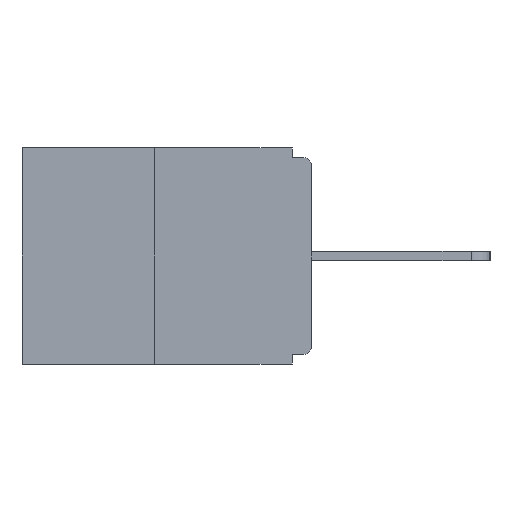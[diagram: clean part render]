
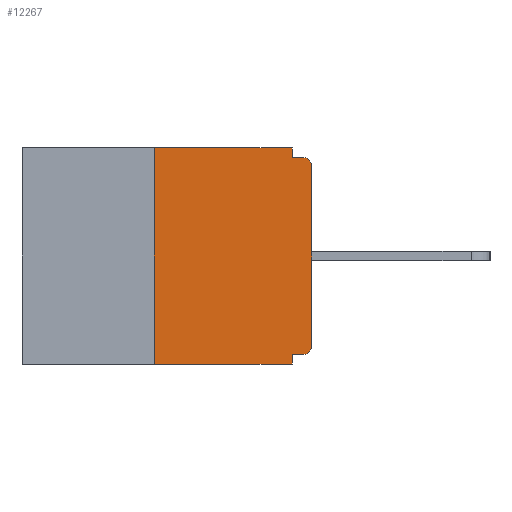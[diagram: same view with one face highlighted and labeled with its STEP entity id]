
A CAD part, left-side view. The second image highlights one B-rep face of the part: STEP entity #12267.
In plain terms, the highlighted planar face has unit normal (-1, 0, 0).
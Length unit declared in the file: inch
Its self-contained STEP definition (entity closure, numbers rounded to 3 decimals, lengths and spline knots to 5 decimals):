
#183 = CARTESIAN_POINT ( 'NONE',  ( 0., 0.031, -0.015 ) ) ;
#197 = VERTEX_POINT ( 'NONE', #6567 ) ;
#548 = PLANE ( 'NONE',  #12446 ) ;
#624 = EDGE_CURVE ( 'NONE', #1537, #197, #9718, .T. ) ;
#679 = CARTESIAN_POINT ( 'NONE',  ( 0., 0.031, -0.328 ) ) ;
#1081 = DIRECTION ( 'NONE',  ( 0., -1., 0. ) ) ;
#1262 = ORIENTED_EDGE ( 'NONE', *, *, #9901, .F. ) ;
#1307 = DIRECTION ( 'NONE',  ( 0., 0., -1. ) ) ;
#1330 = DIRECTION ( 'NONE',  ( -1., 0., 0. ) ) ;
#1537 = VERTEX_POINT ( 'NONE', #15385 ) ;
#1835 = VERTEX_POINT ( 'NONE', #15724 ) ;
#2145 = CARTESIAN_POINT ( 'NONE',  ( 0., 0.25, -0.343 ) ) ;
#2154 = LINE ( 'NONE', #7507, #12647 ) ;
#2473 = CARTESIAN_POINT ( 'NONE',  ( 0., 0.015, -0.03 ) ) ;
#2666 = LINE ( 'NONE', #12496, #3093 ) ;
#2699 = ORIENTED_EDGE ( 'NONE', *, *, #8537, .F. ) ;
#2800 = VERTEX_POINT ( 'NONE', #5422 ) ;
#3093 = VECTOR ( 'NONE', #9903, 39.37008 ) ;
#3209 = DIRECTION ( 'NONE',  ( 0., 0., -1. ) ) ;
#3496 = DIRECTION ( 'NONE',  ( 0., 0., 1. ) ) ;
#3546 = CIRCLE ( 'NONE', #12801, 0.015 ) ;
#3568 = CARTESIAN_POINT ( 'NONE',  ( 0., 0.031, -0.343 ) ) ;
#3932 = DIRECTION ( 'NONE',  ( -1., 0., 0. ) ) ;
#4010 = ORIENTED_EDGE ( 'NONE', *, *, #9820, .F. ) ;
#4133 = ORIENTED_EDGE ( 'NONE', *, *, #13659, .F. ) ;
#4271 = EDGE_CURVE ( 'NONE', #14148, #1537, #15778, .T. ) ;
#4812 = VECTOR ( 'NONE', #1081, 39.37008 ) ;
#4949 = EDGE_LOOP ( 'NONE', ( #2699, #1262, #6456, #15787, #4010, #13012, #8579, #16400, #10294, #4133 ) ) ;
#5394 = VECTOR ( 'NONE', #3496, 39.37008 ) ;
#5422 = CARTESIAN_POINT ( 'NONE',  ( 0., 0.015, -0.328 ) ) ;
#5461 = VECTOR ( 'NONE', #8232, 39.37008 ) ;
#5687 = CARTESIAN_POINT ( 'NONE',  ( 0., 0.46, 0. ) ) ;
#6013 = CARTESIAN_POINT ( 'NONE',  ( 0., 0.25, 0. ) ) ;
#6347 = VERTEX_POINT ( 'NONE', #7987 ) ;
#6456 = ORIENTED_EDGE ( 'NONE', *, *, #12395, .T. ) ;
#6567 = CARTESIAN_POINT ( 'NONE',  ( 0., 0.015, -0.015 ) ) ;
#6991 = VERTEX_POINT ( 'NONE', #6013 ) ;
#7080 = DIRECTION ( 'NONE',  ( 0., -1., 0. ) ) ;
#7507 = CARTESIAN_POINT ( 'NONE',  ( 0., 0.46, -0.343 ) ) ;
#7617 = CARTESIAN_POINT ( 'NONE',  ( 0., 0.031, 0. ) ) ;
#7712 = VERTEX_POINT ( 'NONE', #2145 ) ;
#7987 = CARTESIAN_POINT ( 'NONE',  ( 0., 0.031, -0.343 ) ) ;
#8232 = DIRECTION ( 'NONE',  ( 0., 0., 1. ) ) ;
#8537 = EDGE_CURVE ( 'NONE', #6991, #1835, #15123, .T. ) ;
#8579 = ORIENTED_EDGE ( 'NONE', *, *, #4271, .T. ) ;
#8628 = VECTOR ( 'NONE', #15377, 39.37008 ) ;
#9718 = CIRCLE ( 'NONE', #12404, 0.015 ) ;
#9802 = CARTESIAN_POINT ( 'NONE',  ( 0., 0.46, 0. ) ) ;
#9803 = VECTOR ( 'NONE', #16550, 39.37008 ) ;
#9820 = EDGE_CURVE ( 'NONE', #2800, #10497, #2666, .T. ) ;
#9901 = EDGE_CURVE ( 'NONE', #7712, #6991, #14495, .T. ) ;
#9903 = DIRECTION ( 'NONE',  ( 0., 1., 0. ) ) ;
#10294 = ORIENTED_EDGE ( 'NONE', *, *, #16385, .F. ) ;
#10497 = VERTEX_POINT ( 'NONE', #679 ) ;
#11101 = DIRECTION ( 'NONE',  ( 1., 0., 0. ) ) ;
#11375 = CARTESIAN_POINT ( 'NONE',  ( 0., 0.25, 0. ) ) ;
#11754 = VECTOR ( 'NONE', #7080, 39.37008 ) ;
#11784 = CARTESIAN_POINT ( 'NONE',  ( 0., 0.015, -0.313 ) ) ;
#12267 = ADVANCED_FACE ( 'NONE', ( #12452 ), #548, .F. ) ;
#12395 = EDGE_CURVE ( 'NONE', #7712, #6347, #2154, .T. ) ;
#12404 = AXIS2_PLACEMENT_3D ( 'NONE', #2473, #1330, #1307 ) ;
#12446 = AXIS2_PLACEMENT_3D ( 'NONE', #9802, #11101, #3209 ) ;
#12452 = FACE_OUTER_BOUND ( 'NONE', #4949, .T. ) ;
#12496 = CARTESIAN_POINT ( 'NONE',  ( 0., 0., -0.328 ) ) ;
#12647 = VECTOR ( 'NONE', #15216, 39.37008 ) ;
#12801 = AXIS2_PLACEMENT_3D ( 'NONE', #11784, #3932, #13063 ) ;
#12848 = CARTESIAN_POINT ( 'NONE',  ( 0., 0., -0.015 ) ) ;
#13012 = ORIENTED_EDGE ( 'NONE', *, *, #16480, .T. ) ;
#13063 = DIRECTION ( 'NONE',  ( 0., 0., -1. ) ) ;
#13221 = LINE ( 'NONE', #3568, #9803 ) ;
#13659 = EDGE_CURVE ( 'NONE', #1835, #13883, #15849, .T. ) ;
#13790 = CARTESIAN_POINT ( 'NONE',  ( 0., 0., -0.313 ) ) ;
#13883 = VERTEX_POINT ( 'NONE', #183 ) ;
#14148 = VERTEX_POINT ( 'NONE', #13790 ) ;
#14396 = CARTESIAN_POINT ( 'NONE',  ( 0., 0., 0. ) ) ;
#14495 = LINE ( 'NONE', #11375, #5394 ) ;
#14819 = EDGE_CURVE ( 'NONE', #10497, #6347, #13221, .T. ) ;
#15123 = LINE ( 'NONE', #5687, #11754 ) ;
#15140 = LINE ( 'NONE', #12848, #4812 ) ;
#15216 = DIRECTION ( 'NONE',  ( 0., -1., 0. ) ) ;
#15377 = DIRECTION ( 'NONE',  ( 0., 0., -1. ) ) ;
#15385 = CARTESIAN_POINT ( 'NONE',  ( 0., 0., -0.03 ) ) ;
#15724 = CARTESIAN_POINT ( 'NONE',  ( 0., 0.031, 0. ) ) ;
#15778 = LINE ( 'NONE', #14396, #5461 ) ;
#15787 = ORIENTED_EDGE ( 'NONE', *, *, #14819, .F. ) ;
#15849 = LINE ( 'NONE', #7617, #8628 ) ;
#16385 = EDGE_CURVE ( 'NONE', #13883, #197, #15140, .T. ) ;
#16400 = ORIENTED_EDGE ( 'NONE', *, *, #624, .T. ) ;
#16480 = EDGE_CURVE ( 'NONE', #2800, #14148, #3546, .T. ) ;
#16550 = DIRECTION ( 'NONE',  ( 0., 0., -1. ) ) ;
